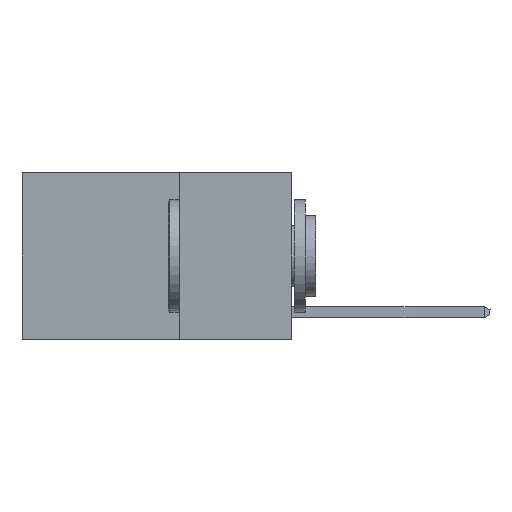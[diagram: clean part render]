
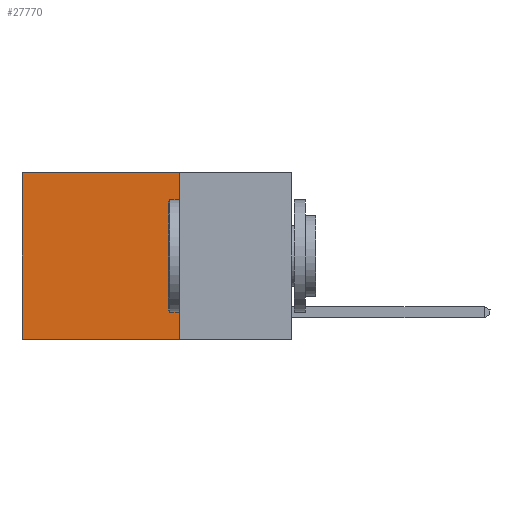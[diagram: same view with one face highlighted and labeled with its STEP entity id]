
A CAD part, left-side view. The second image highlights one B-rep face of the part: STEP entity #27770.
In plain terms, the highlighted planar face has unit normal (-1, 0, 0).
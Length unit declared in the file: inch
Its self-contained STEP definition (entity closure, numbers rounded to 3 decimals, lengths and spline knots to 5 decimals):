
#34 = CARTESIAN_POINT ( 'NONE',  ( 0.2625, 0.25, 0. ) ) ;
#589 = VECTOR ( 'NONE', #8465, 39.37008 ) ;
#1235 = LINE ( 'NONE', #11370, #12469 ) ;
#1561 = AXIS2_PLACEMENT_3D ( 'NONE', #34, #26852, #16053 ) ;
#3512 = VERTEX_POINT ( 'NONE', #28646 ) ;
#4516 = FACE_OUTER_BOUND ( 'NONE', #20091, .T. ) ;
#4919 = ORIENTED_EDGE ( 'NONE', *, *, #15544, .T. ) ;
#7712 = ORIENTED_EDGE ( 'NONE', *, *, #22459, .F. ) ;
#8465 = DIRECTION ( 'NONE',  ( 0., 1., 0. ) ) ;
#9599 = VECTOR ( 'NONE', #25410, 39.37008 ) ;
#10559 = CARTESIAN_POINT ( 'NONE',  ( 0.2625, 0.25, 0. ) ) ;
#11370 = CARTESIAN_POINT ( 'NONE',  ( 0.2625, 0.25, 0. ) ) ;
#12252 = CARTESIAN_POINT ( 'NONE',  ( 0.2625, 0.6, 0. ) ) ;
#12469 = VECTOR ( 'NONE', #20225, 39.37008 ) ;
#15370 = VECTOR ( 'NONE', #16467, 39.37008 ) ;
#15544 = EDGE_CURVE ( 'NONE', #3512, #18890, #21249, .T. ) ;
#16053 = DIRECTION ( 'NONE',  ( 0., 0., -1. ) ) ;
#16083 = EDGE_CURVE ( 'NONE', #22047, #3512, #29000, .T. ) ;
#16269 = CARTESIAN_POINT ( 'NONE',  ( 0.2625, 0.25, -0.37 ) ) ;
#16467 = DIRECTION ( 'NONE',  ( 0., 0., -1. ) ) ;
#18257 = ORIENTED_EDGE ( 'NONE', *, *, #16083, .T. ) ;
#18738 = VERTEX_POINT ( 'NONE', #23538 ) ;
#18890 = VERTEX_POINT ( 'NONE', #26976 ) ;
#20091 = EDGE_LOOP ( 'NONE', ( #4919, #27240, #7712, #18257 ) ) ;
#20225 = DIRECTION ( 'NONE',  ( 0., 0., -1. ) ) ;
#21249 = LINE ( 'NONE', #12252, #15370 ) ;
#22047 = VERTEX_POINT ( 'NONE', #22536 ) ;
#22459 = EDGE_CURVE ( 'NONE', #22047, #18738, #1235, .T. ) ;
#22536 = CARTESIAN_POINT ( 'NONE',  ( 0.2625, 0.25, 0. ) ) ;
#22792 = PLANE ( 'NONE',  #1561 ) ;
#23010 = LINE ( 'NONE', #16269, #9599 ) ;
#23538 = CARTESIAN_POINT ( 'NONE',  ( 0.2625, 0.25, -0.37 ) ) ;
#23928 = EDGE_CURVE ( 'NONE', #18738, #18890, #23010, .T. ) ;
#25410 = DIRECTION ( 'NONE',  ( 0., 1., 0. ) ) ;
#26852 = DIRECTION ( 'NONE',  ( 1., 0., 0. ) ) ;
#26976 = CARTESIAN_POINT ( 'NONE',  ( 0.2625, 0.6, -0.37 ) ) ;
#27240 = ORIENTED_EDGE ( 'NONE', *, *, #23928, .F. ) ;
#27770 = ADVANCED_FACE ( 'NONE', ( #4516 ), #22792, .F. ) ;
#28646 = CARTESIAN_POINT ( 'NONE',  ( 0.2625, 0.6, 0. ) ) ;
#29000 = LINE ( 'NONE', #10559, #589 ) ;
